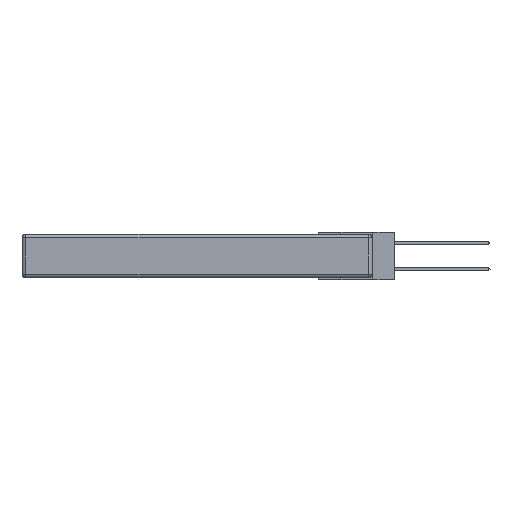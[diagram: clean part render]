
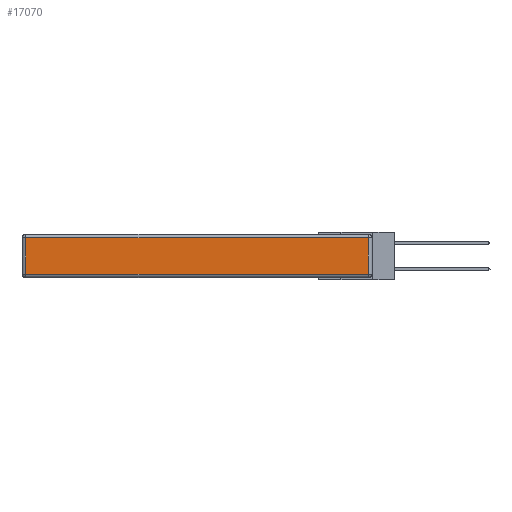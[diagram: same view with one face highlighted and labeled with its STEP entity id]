
A CAD part, left-side view. The second image highlights one B-rep face of the part: STEP entity #17070.
In plain terms, the highlighted planar face has unit normal (-1, 0, 0).
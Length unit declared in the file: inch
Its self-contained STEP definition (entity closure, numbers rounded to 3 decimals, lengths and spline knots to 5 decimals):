
#163 = AXIS2_PLACEMENT_3D ( 'NONE', #11633, #2460, #15903 ) ;
#306 = CARTESIAN_POINT ( 'NONE',  ( 0., 2.72, -0.313 ) ) ;
#726 = PLANE ( 'NONE',  #163 ) ;
#1230 = VECTOR ( 'NONE', #10097, 39.37008 ) ;
#2347 = VERTEX_POINT ( 'NONE', #306 ) ;
#2415 = LINE ( 'NONE', #12894, #4764 ) ;
#2460 = DIRECTION ( 'NONE',  ( -1., 0., 0. ) ) ;
#2744 = EDGE_CURVE ( 'NONE', #16173, #11521, #11571, .T. ) ;
#3093 = ORIENTED_EDGE ( 'NONE', *, *, #19084, .T. ) ;
#4764 = VECTOR ( 'NONE', #14405, 39.37008 ) ;
#6094 = CARTESIAN_POINT ( 'NONE',  ( 0., 0.03, -0.343 ) ) ;
#6659 = VECTOR ( 'NONE', #10782, 39.37008 ) ;
#7134 = LINE ( 'NONE', #6094, #6659 ) ;
#7448 = LINE ( 'NONE', #11918, #1230 ) ;
#7451 = CARTESIAN_POINT ( 'NONE',  ( 0., 2.72, -0.03 ) ) ;
#7860 = CARTESIAN_POINT ( 'NONE',  ( 0., 0.03, -0.313 ) ) ;
#8154 = ORIENTED_EDGE ( 'NONE', *, *, #2744, .T. ) ;
#8594 = ORIENTED_EDGE ( 'NONE', *, *, #14007, .T. ) ;
#9955 = DIRECTION ( 'NONE',  ( 0., 1., 0. ) ) ;
#10097 = DIRECTION ( 'NONE',  ( 0., 0., -1. ) ) ;
#10226 = CARTESIAN_POINT ( 'NONE',  ( 0., 0.03, -0.03 ) ) ;
#10782 = DIRECTION ( 'NONE',  ( 0., 0., 1. ) ) ;
#11334 = EDGE_LOOP ( 'NONE', ( #16946, #3093, #8154, #8594 ) ) ;
#11521 = VERTEX_POINT ( 'NONE', #7451 ) ;
#11571 = LINE ( 'NONE', #14503, #15852 ) ;
#11633 = CARTESIAN_POINT ( 'NONE',  ( 0., 0., -0.343 ) ) ;
#11918 = CARTESIAN_POINT ( 'NONE',  ( 0., 2.72, -0.343 ) ) ;
#12894 = CARTESIAN_POINT ( 'NONE',  ( 0., 0., -0.313 ) ) ;
#14007 = EDGE_CURVE ( 'NONE', #11521, #2347, #7448, .T. ) ;
#14405 = DIRECTION ( 'NONE',  ( 0., -1., 0. ) ) ;
#14503 = CARTESIAN_POINT ( 'NONE',  ( 0., 2.75, -0.03 ) ) ;
#15596 = VERTEX_POINT ( 'NONE', #7860 ) ;
#15852 = VECTOR ( 'NONE', #9955, 39.37008 ) ;
#15903 = DIRECTION ( 'NONE',  ( 0., 0., 1. ) ) ;
#16173 = VERTEX_POINT ( 'NONE', #10226 ) ;
#16946 = ORIENTED_EDGE ( 'NONE', *, *, #17554, .T. ) ;
#17070 = ADVANCED_FACE ( 'NONE', ( #19428 ), #726, .T. ) ;
#17554 = EDGE_CURVE ( 'NONE', #2347, #15596, #2415, .T. ) ;
#19084 = EDGE_CURVE ( 'NONE', #15596, #16173, #7134, .T. ) ;
#19428 = FACE_OUTER_BOUND ( 'NONE', #11334, .T. ) ;
